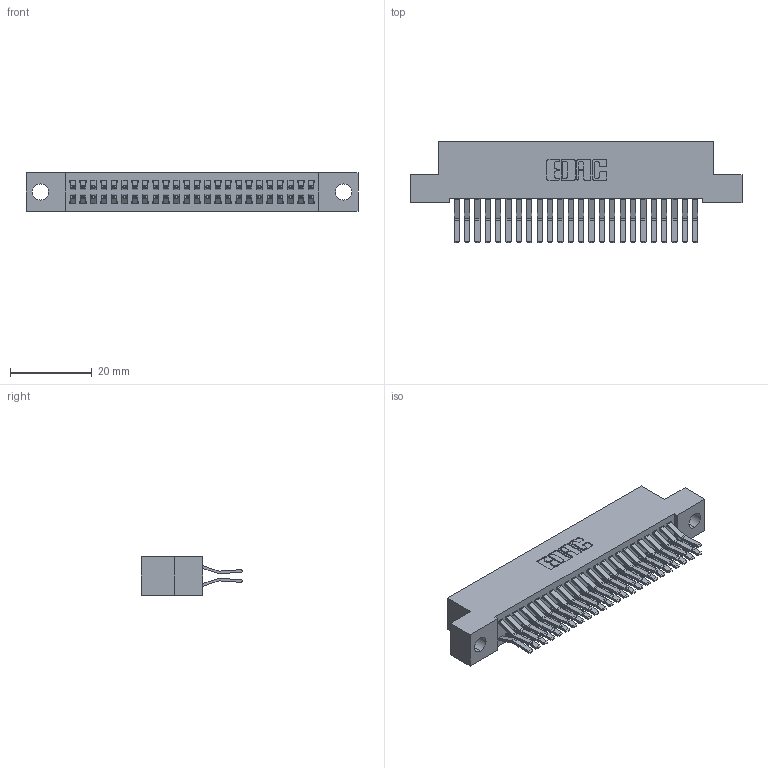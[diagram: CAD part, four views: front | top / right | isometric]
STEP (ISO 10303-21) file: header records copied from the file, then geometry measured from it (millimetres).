
FILE_DESCRIPTION (( 'STEP AP203' ), '1' );
FILE_NAME ('392-048-560-204.STEP', '2019-10-08T01:38:12', ( '' ), ( '' ), 'SwSTEP 2.0', 'SolidWorks 2016', '' );
FILE_SCHEMA (( 'CONFIG_CONTROL_DESIGN' ));
Length unit declared in the file: inch
Products named in the file (3): 392-048-560-204; 342 Part_.156 TH; 345-292-001_560 Tail
Assembly tree (49 placements, depth 2):
  392-048-560-204
    342 Part_.156 TH
    345-292-001_560 Tail  x48
Bounding box: 81.28 x 24.78 x 9.4 mm (x, y, z)
Volume: 7445.9 mm3; surface area: 12256.4 mm2
Topology: 49 solids, 49 shells, 2702 faces, 8027 edges, 5286 vertices
Faces by surface type: plane 1794, cylinder 908
Entity records: 17727 total; most frequent: CARTESIAN_POINT 2958, ORIENTED_EDGE 2894, DIRECTION 2563, EDGE_CURVE 1447, LINE 1315, VECTOR 1315, VERTEX_POINT 962, AXIS2_PLACEMENT_3D 624
